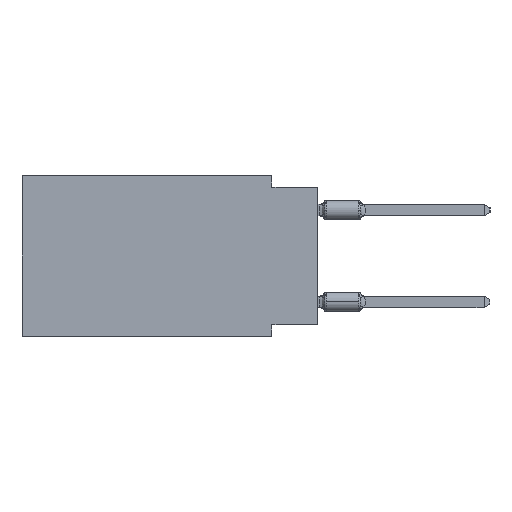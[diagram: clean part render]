
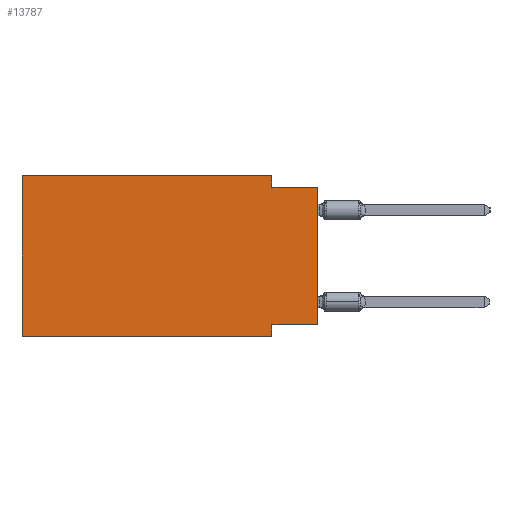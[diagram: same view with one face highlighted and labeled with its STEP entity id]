
A CAD part, left-side view. The second image highlights one B-rep face of the part: STEP entity #13787.
In plain terms, the highlighted planar face has unit normal (-1, 0, 0).
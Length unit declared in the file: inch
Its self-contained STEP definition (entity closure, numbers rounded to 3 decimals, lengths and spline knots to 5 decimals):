
#247 = CARTESIAN_POINT ( 'NONE',  ( 0., 0.645, -0.35 ) ) ;
#337 = LINE ( 'NONE', #18197, #6483 ) ;
#647 = LINE ( 'NONE', #9401, #4269 ) ;
#1174 = VERTEX_POINT ( 'NONE', #11718 ) ;
#1466 = ORIENTED_EDGE ( 'NONE', *, *, #11829, .T. ) ;
#1722 = ORIENTED_EDGE ( 'NONE', *, *, #18231, .F. ) ;
#2807 = DIRECTION ( 'NONE',  ( 0., 0., -1. ) ) ;
#3042 = CARTESIAN_POINT ( 'NONE',  ( 0., 0., -0.025 ) ) ;
#3046 = VECTOR ( 'NONE', #13888, 39.37008 ) ;
#3165 = VERTEX_POINT ( 'NONE', #5159 ) ;
#3547 = DIRECTION ( 'NONE',  ( 0., 0., 1. ) ) ;
#3623 = CARTESIAN_POINT ( 'NONE',  ( 0., 0.1, -0.325 ) ) ;
#4269 = VECTOR ( 'NONE', #18395, 39.37008 ) ;
#4564 = EDGE_CURVE ( 'NONE', #18387, #20450, #12840, .T. ) ;
#4670 = DIRECTION ( 'NONE',  ( 1., 0., 0. ) ) ;
#4716 = VERTEX_POINT ( 'NONE', #10154 ) ;
#4880 = VERTEX_POINT ( 'NONE', #7242 ) ;
#5159 = CARTESIAN_POINT ( 'NONE',  ( 0., 0.1, -0.35 ) ) ;
#5267 = LINE ( 'NONE', #12153, #3046 ) ;
#5734 = CARTESIAN_POINT ( 'NONE',  ( 0., 0.645, 0. ) ) ;
#6153 = VERTEX_POINT ( 'NONE', #19731 ) ;
#6328 = DIRECTION ( 'NONE',  ( 0., -1., 0. ) ) ;
#6483 = VECTOR ( 'NONE', #21824, 39.37008 ) ;
#7196 = CARTESIAN_POINT ( 'NONE',  ( 0., 0., 0. ) ) ;
#7242 = CARTESIAN_POINT ( 'NONE',  ( 0., 0.1, 0. ) ) ;
#7620 = LINE ( 'NONE', #7196, #9334 ) ;
#8188 = VECTOR ( 'NONE', #6328, 39.37008 ) ;
#8202 = FACE_OUTER_BOUND ( 'NONE', #8996, .T. ) ;
#8522 = VERTEX_POINT ( 'NONE', #3623 ) ;
#8996 = EDGE_LOOP ( 'NONE', ( #19484, #1722, #13179, #21378, #14708, #1466, #15139, #12880 ) ) ;
#9334 = VECTOR ( 'NONE', #3547, 39.37008 ) ;
#9355 = DIRECTION ( 'NONE',  ( 0., 0., 1. ) ) ;
#9401 = CARTESIAN_POINT ( 'NONE',  ( 0., 0.645, -0.35 ) ) ;
#10154 = CARTESIAN_POINT ( 'NONE',  ( 0., 0., -0.325 ) ) ;
#10755 = CARTESIAN_POINT ( 'NONE',  ( 0., 0., -0.325 ) ) ;
#11018 = EDGE_CURVE ( 'NONE', #20450, #4880, #337, .T. ) ;
#11718 = CARTESIAN_POINT ( 'NONE',  ( 0., 0., -0.025 ) ) ;
#11821 = LINE ( 'NONE', #3042, #8188 ) ;
#11829 = EDGE_CURVE ( 'NONE', #18387, #3165, #647, .T. ) ;
#12153 = CARTESIAN_POINT ( 'NONE',  ( 0., 0.1, 0. ) ) ;
#12840 = LINE ( 'NONE', #5734, #13978 ) ;
#12880 = ORIENTED_EDGE ( 'NONE', *, *, #13601, .F. ) ;
#13179 = ORIENTED_EDGE ( 'NONE', *, *, #21677, .F. ) ;
#13434 = LINE ( 'NONE', #16956, #14168 ) ;
#13601 = EDGE_CURVE ( 'NONE', #4716, #8522, #21524, .T. ) ;
#13787 = ADVANCED_FACE ( 'NONE', ( #8202 ), #22331, .F. ) ;
#13888 = DIRECTION ( 'NONE',  ( 0., 0., -1. ) ) ;
#13978 = VECTOR ( 'NONE', #9355, 39.37008 ) ;
#14168 = VECTOR ( 'NONE', #2807, 39.37008 ) ;
#14708 = ORIENTED_EDGE ( 'NONE', *, *, #4564, .F. ) ;
#14935 = EDGE_CURVE ( 'NONE', #4716, #1174, #7620, .T. ) ;
#15003 = EDGE_CURVE ( 'NONE', #8522, #3165, #13434, .T. ) ;
#15139 = ORIENTED_EDGE ( 'NONE', *, *, #15003, .F. ) ;
#15313 = CARTESIAN_POINT ( 'NONE',  ( 0., 0.645, 0. ) ) ;
#15428 = DIRECTION ( 'NONE',  ( 0., 0., -1. ) ) ;
#16643 = VECTOR ( 'NONE', #21297, 39.37008 ) ;
#16956 = CARTESIAN_POINT ( 'NONE',  ( 0., 0.1, -0.35 ) ) ;
#18197 = CARTESIAN_POINT ( 'NONE',  ( 0., 0.645, 0. ) ) ;
#18231 = EDGE_CURVE ( 'NONE', #6153, #1174, #11821, .T. ) ;
#18387 = VERTEX_POINT ( 'NONE', #247 ) ;
#18395 = DIRECTION ( 'NONE',  ( 0., -1., 0. ) ) ;
#19484 = ORIENTED_EDGE ( 'NONE', *, *, #14935, .T. ) ;
#19731 = CARTESIAN_POINT ( 'NONE',  ( 0., 0.1, -0.025 ) ) ;
#20294 = AXIS2_PLACEMENT_3D ( 'NONE', #15313, #4670, #15428 ) ;
#20450 = VERTEX_POINT ( 'NONE', #22316 ) ;
#21297 = DIRECTION ( 'NONE',  ( 0., 1., 0. ) ) ;
#21378 = ORIENTED_EDGE ( 'NONE', *, *, #11018, .F. ) ;
#21524 = LINE ( 'NONE', #10755, #16643 ) ;
#21677 = EDGE_CURVE ( 'NONE', #4880, #6153, #5267, .T. ) ;
#21824 = DIRECTION ( 'NONE',  ( 0., -1., 0. ) ) ;
#22316 = CARTESIAN_POINT ( 'NONE',  ( 0., 0.645, 0. ) ) ;
#22331 = PLANE ( 'NONE',  #20294 ) ;
